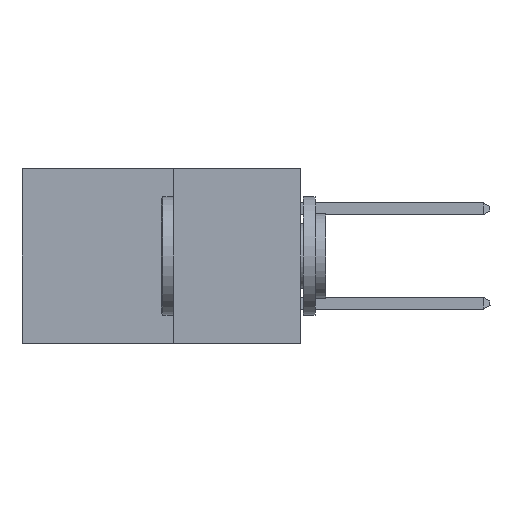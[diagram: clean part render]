
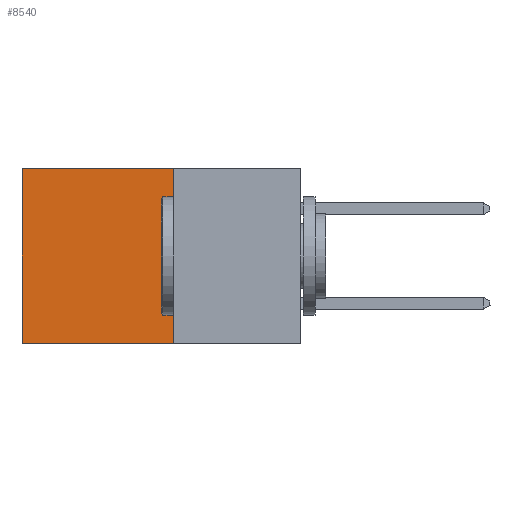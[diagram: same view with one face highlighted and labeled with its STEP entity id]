
A CAD part, left-side view. The second image highlights one B-rep face of the part: STEP entity #8540.
In plain terms, the highlighted planar face has unit normal (-1, 0, 0).
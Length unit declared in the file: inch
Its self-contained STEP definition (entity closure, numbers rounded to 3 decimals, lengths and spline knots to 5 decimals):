
#324 = VERTEX_POINT ( 'NONE', #408 ) ;
#408 = CARTESIAN_POINT ( 'NONE',  ( 0.277, 0.59, 0. ) ) ;
#488 = DIRECTION ( 'NONE',  ( 0., 0., -1. ) ) ;
#1349 = DIRECTION ( 'NONE',  ( 0., 0., -1. ) ) ;
#1661 = VERTEX_POINT ( 'NONE', #7636 ) ;
#1742 = FACE_OUTER_BOUND ( 'NONE', #3366, .T. ) ;
#2495 = VECTOR ( 'NONE', #1349, 39.37008 ) ;
#3296 = CARTESIAN_POINT ( 'NONE',  ( 0.277, 0.27, 0. ) ) ;
#3366 = EDGE_LOOP ( 'NONE', ( #14592, #5847, #6139, #13035 ) ) ;
#3510 = EDGE_CURVE ( 'NONE', #6227, #9215, #8725, .T. ) ;
#4063 = PLANE ( 'NONE',  #6030 ) ;
#4945 = CARTESIAN_POINT ( 'NONE',  ( 0.277, 0.59, -0.37 ) ) ;
#4946 = LINE ( 'NONE', #4945, #2495 ) ;
#5210 = CARTESIAN_POINT ( 'NONE',  ( 0.277, 0.27, -0.37 ) ) ;
#5297 = DIRECTION ( 'NONE',  ( 1., 0., 0. ) ) ;
#5847 = ORIENTED_EDGE ( 'NONE', *, *, #3510, .F. ) ;
#6030 = AXIS2_PLACEMENT_3D ( 'NONE', #12590, #5297, #13820 ) ;
#6139 = ORIENTED_EDGE ( 'NONE', *, *, #9220, .F. ) ;
#6227 = VERTEX_POINT ( 'NONE', #5210 ) ;
#6539 = CARTESIAN_POINT ( 'NONE',  ( 0.277, 0.59, -0.37 ) ) ;
#7627 = CARTESIAN_POINT ( 'NONE',  ( 0.277, 0.27, -0.37 ) ) ;
#7636 = CARTESIAN_POINT ( 'NONE',  ( 0.277, 0.27, 0. ) ) ;
#8516 = VECTOR ( 'NONE', #14187, 39.37008 ) ;
#8540 = ADVANCED_FACE ( 'NONE', ( #1742 ), #4063, .F. ) ;
#8725 = LINE ( 'NONE', #7627, #14821 ) ;
#9215 = VERTEX_POINT ( 'NONE', #6539 ) ;
#9220 = EDGE_CURVE ( 'NONE', #1661, #6227, #13356, .T. ) ;
#10099 = VECTOR ( 'NONE', #488, 39.37008 ) ;
#11583 = EDGE_CURVE ( 'NONE', #1661, #324, #11753, .T. ) ;
#11753 = LINE ( 'NONE', #3296, #8516 ) ;
#12590 = CARTESIAN_POINT ( 'NONE',  ( 0.277, 0.27, -0.37 ) ) ;
#13035 = ORIENTED_EDGE ( 'NONE', *, *, #11583, .T. ) ;
#13356 = LINE ( 'NONE', #15056, #10099 ) ;
#13820 = DIRECTION ( 'NONE',  ( 0., 0., -1. ) ) ;
#13937 = DIRECTION ( 'NONE',  ( 0., 1., 0. ) ) ;
#14187 = DIRECTION ( 'NONE',  ( 0., 1., 0. ) ) ;
#14513 = EDGE_CURVE ( 'NONE', #324, #9215, #4946, .T. ) ;
#14592 = ORIENTED_EDGE ( 'NONE', *, *, #14513, .T. ) ;
#14821 = VECTOR ( 'NONE', #13937, 39.37008 ) ;
#15056 = CARTESIAN_POINT ( 'NONE',  ( 0.277, 0.27, -0.37 ) ) ;
